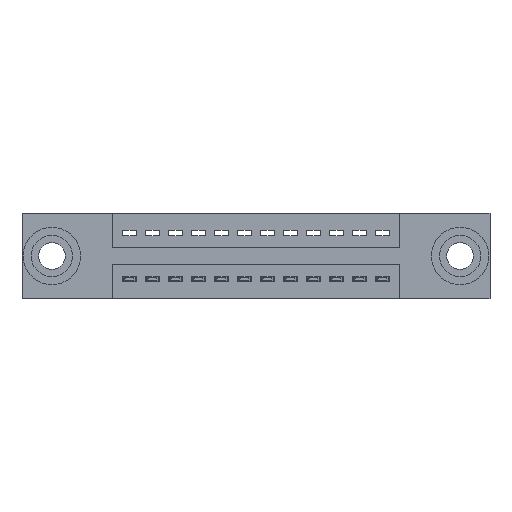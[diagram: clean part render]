
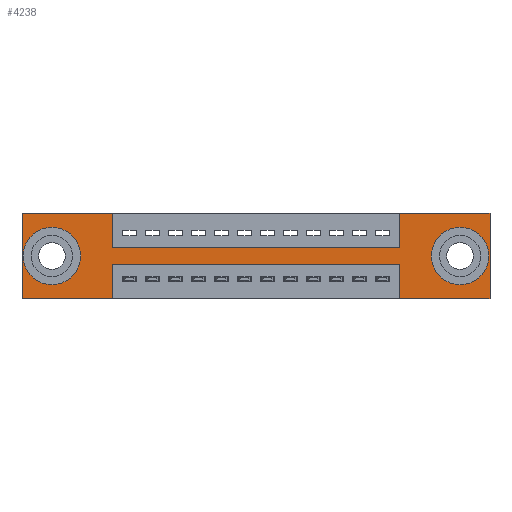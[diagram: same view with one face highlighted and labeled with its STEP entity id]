
A CAD part, front view. The second image highlights one B-rep face of the part: STEP entity #4238.
In plain terms, the highlighted planar face has unit normal (0, -1, 0).
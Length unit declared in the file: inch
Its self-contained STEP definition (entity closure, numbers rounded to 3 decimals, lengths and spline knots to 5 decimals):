
#145 = DIRECTION ( 'NONE',  ( 0., 1., 0. ) ) ;
#311 = FACE_BOUND ( 'NONE', #4553, .T. ) ;
#608 = CARTESIAN_POINT ( 'NONE',  ( 0.3925, 0., 0. ) ) ;
#682 = DIRECTION ( 'NONE',  ( 0., 0., 1. ) ) ;
#709 = VERTEX_POINT ( 'NONE', #7150 ) ;
#763 = DIRECTION ( 'NONE',  ( -1., 0., 0. ) ) ;
#776 = DIRECTION ( 'NONE',  ( 0., 0., -1. ) ) ;
#824 = CARTESIAN_POINT ( 'NONE',  ( 0., 0., 0. ) ) ;
#964 = ORIENTED_EDGE ( 'NONE', *, *, #9962, .F. ) ;
#1131 = LINE ( 'NONE', #5129, #9442 ) ;
#1140 = EDGE_CURVE ( 'NONE', #8001, #7413, #13167, .T. ) ;
#1167 = CARTESIAN_POINT ( 'NONE',  ( 1.905, 0., -0.185 ) ) ;
#1232 = VERTEX_POINT ( 'NONE', #2823 ) ;
#1355 = VERTEX_POINT ( 'NONE', #13555 ) ;
#1474 = ORIENTED_EDGE ( 'NONE', *, *, #7232, .F. ) ;
#1495 = CARTESIAN_POINT ( 'NONE',  ( 0.13, 0., -0.185 ) ) ;
#1567 = PLANE ( 'NONE',  #4244 ) ;
#1579 = CIRCLE ( 'NONE', #8468, 0.078 ) ;
#1978 = CARTESIAN_POINT ( 'NONE',  ( 0.3925, 0., -0.22 ) ) ;
#1981 = EDGE_CURVE ( 'NONE', #11641, #709, #6594, .T. ) ;
#2065 = DIRECTION ( 'NONE',  ( -1., 0., 0. ) ) ;
#2091 = DIRECTION ( 'NONE',  ( 1., 0., 0. ) ) ;
#2164 = VECTOR ( 'NONE', #763, 39.37008 ) ;
#2423 = DIRECTION ( 'NONE',  ( 0., 1., 0. ) ) ;
#2467 = DIRECTION ( 'NONE',  ( 0., 0., 1. ) ) ;
#2485 = DIRECTION ( 'NONE',  ( 0., -1., 0. ) ) ;
#2659 = CARTESIAN_POINT ( 'NONE',  ( 1.6425, 0., 0. ) ) ;
#2702 = DIRECTION ( 'NONE',  ( 0., 0., -1. ) ) ;
#2715 = VECTOR ( 'NONE', #4788, 39.37008 ) ;
#2823 = CARTESIAN_POINT ( 'NONE',  ( 2.035, 0., 0. ) ) ;
#3019 = ORIENTED_EDGE ( 'NONE', *, *, #12385, .F. ) ;
#3065 = VECTOR ( 'NONE', #2065, 39.37008 ) ;
#3074 = CARTESIAN_POINT ( 'NONE',  ( 0., 0., 0. ) ) ;
#3304 = CARTESIAN_POINT ( 'NONE',  ( 0.3925, 0., -0.37 ) ) ;
#3536 = EDGE_CURVE ( 'NONE', #9083, #8001, #8516, .T. ) ;
#3581 = VECTOR ( 'NONE', #9364, 39.37008 ) ;
#3590 = ORIENTED_EDGE ( 'NONE', *, *, #8543, .F. ) ;
#3713 = CARTESIAN_POINT ( 'NONE',  ( 0., 0., -0.37 ) ) ;
#3797 = CARTESIAN_POINT ( 'NONE',  ( 0., 0., 0. ) ) ;
#3921 = LINE ( 'NONE', #6084, #7485 ) ;
#4024 = VECTOR ( 'NONE', #8095, 39.37008 ) ;
#4213 = ORIENTED_EDGE ( 'NONE', *, *, #6021, .T. ) ;
#4238 = ADVANCED_FACE ( 'NONE', ( #8800, #311, #9450 ), #1567, .T. ) ;
#4240 = EDGE_LOOP ( 'NONE', ( #10929, #13234 ) ) ;
#4244 = AXIS2_PLACEMENT_3D ( 'NONE', #13013, #2485, #5578 ) ;
#4300 = AXIS2_PLACEMENT_3D ( 'NONE', #12144, #9085, #776 ) ;
#4459 = CARTESIAN_POINT ( 'NONE',  ( 1.6425, 0., 0. ) ) ;
#4533 = ORIENTED_EDGE ( 'NONE', *, *, #1140, .F. ) ;
#4553 = EDGE_LOOP ( 'NONE', ( #11918, #4213 ) ) ;
#4582 = CIRCLE ( 'NONE', #10348, 0.078 ) ;
#4761 = DIRECTION ( 'NONE',  ( -1., 0., 0. ) ) ;
#4788 = DIRECTION ( 'NONE',  ( 1., 0., 0. ) ) ;
#5129 = CARTESIAN_POINT ( 'NONE',  ( 0.3925, 0., -0.37 ) ) ;
#5186 = VERTEX_POINT ( 'NONE', #7697 ) ;
#5387 = DIRECTION ( 'NONE',  ( 0., 0., -1. ) ) ;
#5578 = DIRECTION ( 'NONE',  ( 0., 0., -1. ) ) ;
#5617 = EDGE_LOOP ( 'NONE', ( #1474, #3019, #3590, #10451, #13421, #7727, #964, #8509, #12603, #10007, #4533, #12689 ) ) ;
#5619 = AXIS2_PLACEMENT_3D ( 'NONE', #1167, #145, #5387 ) ;
#6021 = EDGE_CURVE ( 'NONE', #9916, #12819, #4582, .T. ) ;
#6084 = CARTESIAN_POINT ( 'NONE',  ( 2.035, 0., 0. ) ) ;
#6136 = LINE ( 'NONE', #3797, #2715 ) ;
#6540 = EDGE_CURVE ( 'NONE', #6884, #5186, #9439, .T. ) ;
#6594 = CIRCLE ( 'NONE', #5619, 0.078 ) ;
#6767 = CARTESIAN_POINT ( 'NONE',  ( 1.905, 0., -0.263 ) ) ;
#6884 = VERTEX_POINT ( 'NONE', #608 ) ;
#7047 = DIRECTION ( 'NONE',  ( 0., 0., -1. ) ) ;
#7055 = EDGE_CURVE ( 'NONE', #1232, #11300, #3921, .T. ) ;
#7150 = CARTESIAN_POINT ( 'NONE',  ( 1.905, 0., -0.107 ) ) ;
#7232 = EDGE_CURVE ( 'NONE', #7995, #9083, #1131, .T. ) ;
#7413 = VERTEX_POINT ( 'NONE', #3074 ) ;
#7480 = VERTEX_POINT ( 'NONE', #4459 ) ;
#7485 = VECTOR ( 'NONE', #7047, 39.37008 ) ;
#7492 = CIRCLE ( 'NONE', #4300, 0.078 ) ;
#7582 = VECTOR ( 'NONE', #10109, 39.37008 ) ;
#7697 = CARTESIAN_POINT ( 'NONE',  ( 0.3925, 0., -0.15 ) ) ;
#7727 = ORIENTED_EDGE ( 'NONE', *, *, #13319, .F. ) ;
#7906 = LINE ( 'NONE', #2659, #7582 ) ;
#7934 = CARTESIAN_POINT ( 'NONE',  ( 0.3925, 0., 0. ) ) ;
#7995 = VERTEX_POINT ( 'NONE', #10747 ) ;
#8000 = CARTESIAN_POINT ( 'NONE',  ( 0., 0., -0.37 ) ) ;
#8001 = VERTEX_POINT ( 'NONE', #3713 ) ;
#8068 = CARTESIAN_POINT ( 'NONE',  ( 1.6425, 0., -0.22 ) ) ;
#8095 = DIRECTION ( 'NONE',  ( 1., 0., 0. ) ) ;
#8123 = LINE ( 'NONE', #12489, #3581 ) ;
#8130 = LINE ( 'NONE', #1978, #3065 ) ;
#8155 = VECTOR ( 'NONE', #4761, 39.37008 ) ;
#8291 = CARTESIAN_POINT ( 'NONE',  ( 0.3925, 0., -0.15 ) ) ;
#8426 = VECTOR ( 'NONE', #682, 39.37008 ) ;
#8468 = AXIS2_PLACEMENT_3D ( 'NONE', #1495, #2423, #2467 ) ;
#8509 = ORIENTED_EDGE ( 'NONE', *, *, #12813, .F. ) ;
#8516 = LINE ( 'NONE', #9155, #2164 ) ;
#8543 = EDGE_CURVE ( 'NONE', #1355, #10549, #8123, .T. ) ;
#8633 = VECTOR ( 'NONE', #2702, 39.37008 ) ;
#8800 = FACE_BOUND ( 'NONE', #4240, .T. ) ;
#8802 = EDGE_CURVE ( 'NONE', #12819, #9916, #1579, .T. ) ;
#9064 = LINE ( 'NONE', #824, #4024 ) ;
#9083 = VERTEX_POINT ( 'NONE', #3304 ) ;
#9085 = DIRECTION ( 'NONE',  ( 0., 1., 0. ) ) ;
#9155 = CARTESIAN_POINT ( 'NONE',  ( 0., 0., -0.37 ) ) ;
#9181 = VERTEX_POINT ( 'NONE', #10380 ) ;
#9271 = CARTESIAN_POINT ( 'NONE',  ( 0.13, 0., -0.107 ) ) ;
#9364 = DIRECTION ( 'NONE',  ( 0., 0., 1. ) ) ;
#9400 = EDGE_CURVE ( 'NONE', #7413, #6884, #6136, .T. ) ;
#9439 = LINE ( 'NONE', #7934, #8633 ) ;
#9442 = VECTOR ( 'NONE', #13513, 39.37008 ) ;
#9450 = FACE_OUTER_BOUND ( 'NONE', #5617, .T. ) ;
#9916 = VERTEX_POINT ( 'NONE', #10561 ) ;
#9962 = EDGE_CURVE ( 'NONE', #9181, #7480, #7906, .T. ) ;
#10007 = ORIENTED_EDGE ( 'NONE', *, *, #9400, .F. ) ;
#10063 = VECTOR ( 'NONE', #2091, 39.37008 ) ;
#10109 = DIRECTION ( 'NONE',  ( 0., 0., 1. ) ) ;
#10154 = CARTESIAN_POINT ( 'NONE',  ( 0., 0., 0. ) ) ;
#10348 = AXIS2_PLACEMENT_3D ( 'NONE', #11217, #11304, #12368 ) ;
#10380 = CARTESIAN_POINT ( 'NONE',  ( 1.6425, 0., -0.15 ) ) ;
#10451 = ORIENTED_EDGE ( 'NONE', *, *, #11251, .F. ) ;
#10549 = VERTEX_POINT ( 'NONE', #8068 ) ;
#10561 = CARTESIAN_POINT ( 'NONE',  ( 0.13, 0., -0.263 ) ) ;
#10747 = CARTESIAN_POINT ( 'NONE',  ( 0.3925, 0., -0.22 ) ) ;
#10906 = LINE ( 'NONE', #8000, #8155 ) ;
#10929 = ORIENTED_EDGE ( 'NONE', *, *, #11248, .T. ) ;
#11217 = CARTESIAN_POINT ( 'NONE',  ( 0.13, 0., -0.185 ) ) ;
#11248 = EDGE_CURVE ( 'NONE', #709, #11641, #7492, .T. ) ;
#11251 = EDGE_CURVE ( 'NONE', #11300, #1355, #10906, .T. ) ;
#11300 = VERTEX_POINT ( 'NONE', #13090 ) ;
#11304 = DIRECTION ( 'NONE',  ( 0., 1., 0. ) ) ;
#11511 = LINE ( 'NONE', #8291, #10063 ) ;
#11641 = VERTEX_POINT ( 'NONE', #6767 ) ;
#11918 = ORIENTED_EDGE ( 'NONE', *, *, #8802, .T. ) ;
#12144 = CARTESIAN_POINT ( 'NONE',  ( 1.905, 0., -0.185 ) ) ;
#12368 = DIRECTION ( 'NONE',  ( 0., 0., 1. ) ) ;
#12385 = EDGE_CURVE ( 'NONE', #10549, #7995, #8130, .T. ) ;
#12489 = CARTESIAN_POINT ( 'NONE',  ( 1.6425, 0., -0.37 ) ) ;
#12603 = ORIENTED_EDGE ( 'NONE', *, *, #6540, .F. ) ;
#12689 = ORIENTED_EDGE ( 'NONE', *, *, #3536, .F. ) ;
#12813 = EDGE_CURVE ( 'NONE', #5186, #9181, #11511, .T. ) ;
#12819 = VERTEX_POINT ( 'NONE', #9271 ) ;
#13013 = CARTESIAN_POINT ( 'NONE',  ( 0., 0., -0.37 ) ) ;
#13090 = CARTESIAN_POINT ( 'NONE',  ( 2.035, 0., -0.37 ) ) ;
#13167 = LINE ( 'NONE', #10154, #8426 ) ;
#13234 = ORIENTED_EDGE ( 'NONE', *, *, #1981, .T. ) ;
#13319 = EDGE_CURVE ( 'NONE', #7480, #1232, #9064, .T. ) ;
#13421 = ORIENTED_EDGE ( 'NONE', *, *, #7055, .F. ) ;
#13513 = DIRECTION ( 'NONE',  ( 0., 0., -1. ) ) ;
#13555 = CARTESIAN_POINT ( 'NONE',  ( 1.6425, 0., -0.37 ) ) ;
